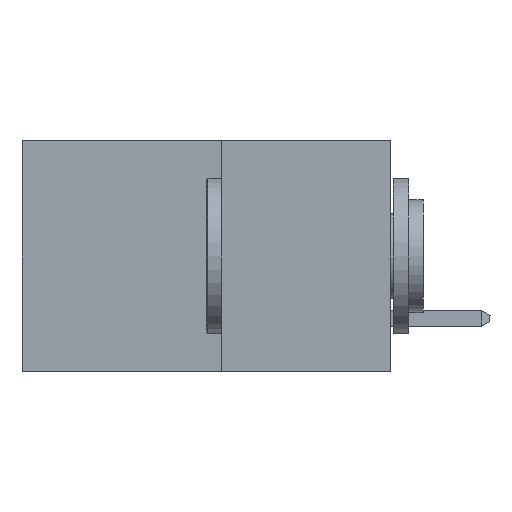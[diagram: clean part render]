
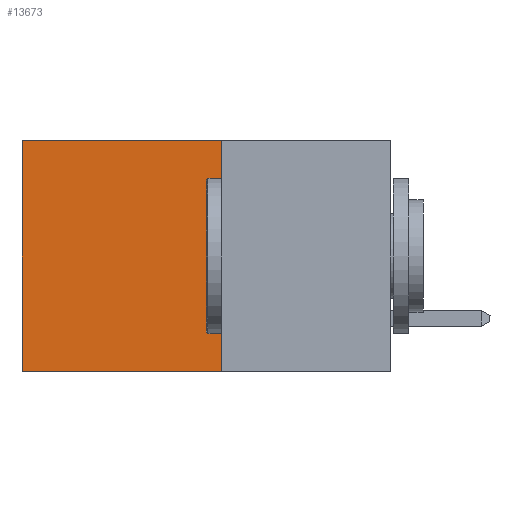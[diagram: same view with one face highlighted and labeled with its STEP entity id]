
A CAD part, left-side view. The second image highlights one B-rep face of the part: STEP entity #13673.
In plain terms, the highlighted planar face has unit normal (-1, 0, 0).
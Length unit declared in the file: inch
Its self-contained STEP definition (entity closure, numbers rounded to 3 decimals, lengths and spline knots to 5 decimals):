
#338 = EDGE_CURVE ( 'NONE', #21807, #29992, #14630, .T. ) ;
#1070 = CARTESIAN_POINT ( 'NONE',  ( 0.277, 0.27, -0.37 ) ) ;
#2711 = LINE ( 'NONE', #10894, #8317 ) ;
#6255 = DIRECTION ( 'NONE',  ( 0., 0., -1. ) ) ;
#6909 = DIRECTION ( 'NONE',  ( 1., 0., 0. ) ) ;
#7049 = PLANE ( 'NONE',  #14538 ) ;
#7123 = FACE_OUTER_BOUND ( 'NONE', #25691, .T. ) ;
#7742 = CARTESIAN_POINT ( 'NONE',  ( 0.277, 0.27, -0.37 ) ) ;
#7951 = DIRECTION ( 'NONE',  ( 0., 0., -1. ) ) ;
#8317 = VECTOR ( 'NONE', #22784, 39.37008 ) ;
#8945 = VECTOR ( 'NONE', #10030, 39.37008 ) ;
#9718 = LINE ( 'NONE', #15867, #8945 ) ;
#10030 = DIRECTION ( 'NONE',  ( 0., 1., 0. ) ) ;
#10894 = CARTESIAN_POINT ( 'NONE',  ( 0.277, 0.27, -0.37 ) ) ;
#11374 = VERTEX_POINT ( 'NONE', #13179 ) ;
#13179 = CARTESIAN_POINT ( 'NONE',  ( 0.277, 0.59, 0. ) ) ;
#13594 = VECTOR ( 'NONE', #24479, 39.37008 ) ;
#13673 = ADVANCED_FACE ( 'NONE', ( #7123 ), #7049, .F. ) ;
#14538 = AXIS2_PLACEMENT_3D ( 'NONE', #7742, #6909, #6255 ) ;
#14630 = LINE ( 'NONE', #16956, #15385 ) ;
#15385 = VECTOR ( 'NONE', #7951, 39.37008 ) ;
#15867 = CARTESIAN_POINT ( 'NONE',  ( 0.277, 0.27, 0. ) ) ;
#16387 = ORIENTED_EDGE ( 'NONE', *, *, #338, .F. ) ;
#16956 = CARTESIAN_POINT ( 'NONE',  ( 0.277, 0.27, -0.37 ) ) ;
#17295 = EDGE_CURVE ( 'NONE', #11374, #29346, #26061, .T. ) ;
#18546 = ORIENTED_EDGE ( 'NONE', *, *, #17295, .T. ) ;
#19126 = EDGE_CURVE ( 'NONE', #21807, #11374, #9718, .T. ) ;
#21807 = VERTEX_POINT ( 'NONE', #28014 ) ;
#22537 = CARTESIAN_POINT ( 'NONE',  ( 0.277, 0.59, -0.37 ) ) ;
#22784 = DIRECTION ( 'NONE',  ( 0., 1., 0. ) ) ;
#23965 = ORIENTED_EDGE ( 'NONE', *, *, #26584, .F. ) ;
#24441 = CARTESIAN_POINT ( 'NONE',  ( 0.277, 0.59, -0.37 ) ) ;
#24479 = DIRECTION ( 'NONE',  ( 0., 0., -1. ) ) ;
#25236 = ORIENTED_EDGE ( 'NONE', *, *, #19126, .T. ) ;
#25691 = EDGE_LOOP ( 'NONE', ( #18546, #23965, #16387, #25236 ) ) ;
#26061 = LINE ( 'NONE', #24441, #13594 ) ;
#26584 = EDGE_CURVE ( 'NONE', #29992, #29346, #2711, .T. ) ;
#28014 = CARTESIAN_POINT ( 'NONE',  ( 0.277, 0.27, 0. ) ) ;
#29346 = VERTEX_POINT ( 'NONE', #22537 ) ;
#29992 = VERTEX_POINT ( 'NONE', #1070 ) ;
